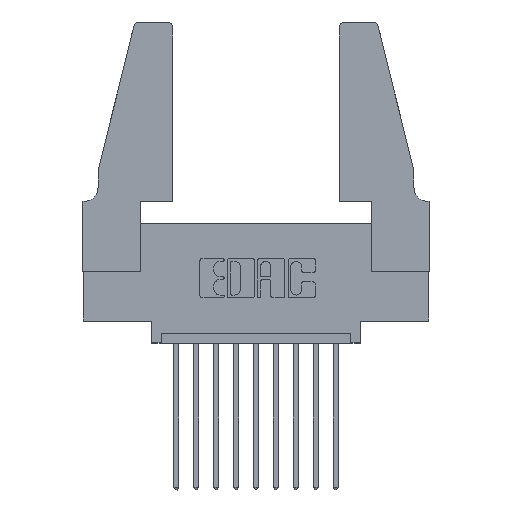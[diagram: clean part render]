
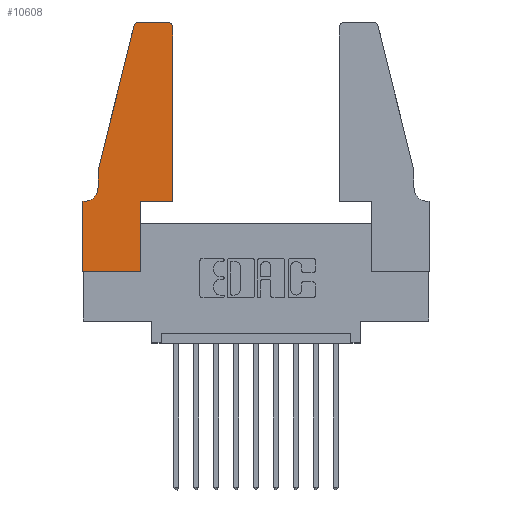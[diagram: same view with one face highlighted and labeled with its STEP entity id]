
A CAD part, top view. The second image highlights one B-rep face of the part: STEP entity #10608.
In plain terms, the highlighted planar face has unit normal (0, 0, 1).
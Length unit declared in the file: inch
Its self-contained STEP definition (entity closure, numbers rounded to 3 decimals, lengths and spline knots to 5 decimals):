
#60 = LINE ( 'NONE', #7379, #5006 ) ;
#385 = CARTESIAN_POINT ( 'NONE',  ( 0.0055, 0.42, 0.37 ) ) ;
#438 = DIRECTION ( 'NONE',  ( 0., -1., 0. ) ) ;
#533 = LINE ( 'NONE', #12607, #9063 ) ;
#755 = ORIENTED_EDGE ( 'NONE', *, *, #12746, .T. ) ;
#870 = LINE ( 'NONE', #3170, #8243 ) ;
#896 = CIRCLE ( 'NONE', #7988, 0.03 ) ;
#925 = CARTESIAN_POINT ( 'NONE',  ( 0.0755, 0.5, 0.37 ) ) ;
#957 = EDGE_CURVE ( 'NONE', #6256, #11347, #60, .T. ) ;
#1126 = AXIS2_PLACEMENT_3D ( 'NONE', #10207, #1919, #12230 ) ;
#1200 = EDGE_CURVE ( 'NONE', #6721, #6256, #12847, .T. ) ;
#1493 = VERTEX_POINT ( 'NONE', #5527 ) ;
#1587 = CARTESIAN_POINT ( 'NONE',  ( 0.2865, 0.35, 0.37 ) ) ;
#1686 = EDGE_CURVE ( 'NONE', #3656, #1854, #870, .T. ) ;
#1854 = VERTEX_POINT ( 'NONE', #8184 ) ;
#1919 = DIRECTION ( 'NONE',  ( 0., 0., 1. ) ) ;
#2016 = ORIENTED_EDGE ( 'NONE', *, *, #1200, .T. ) ;
#2304 = DIRECTION ( 'NONE',  ( 0., 1., 0. ) ) ;
#2331 = CARTESIAN_POINT ( 'NONE',  ( 0., 0.35, 0.37 ) ) ;
#2590 = CARTESIAN_POINT ( 'NONE',  ( 0.4505, 0.35, 0.37 ) ) ;
#2625 = DIRECTION ( 'NONE',  ( 0., 0., 1. ) ) ;
#2951 = AXIS2_PLACEMENT_3D ( 'NONE', #2331, #11775, #6443 ) ;
#2980 = LINE ( 'NONE', #12002, #6935 ) ;
#3170 = CARTESIAN_POINT ( 'NONE',  ( 0.2605, 1.25, 0.37 ) ) ;
#3343 = CIRCLE ( 'NONE', #1126, 0.03 ) ;
#3351 = DIRECTION ( 'NONE',  ( 1., 0., 0. ) ) ;
#3488 = CARTESIAN_POINT ( 'NONE',  ( 0.0755, 0.42, 0.37 ) ) ;
#3578 = VERTEX_POINT ( 'NONE', #925 ) ;
#3620 = ORIENTED_EDGE ( 'NONE', *, *, #957, .T. ) ;
#3642 = VERTEX_POINT ( 'NONE', #6385 ) ;
#3656 = VERTEX_POINT ( 'NONE', #6252 ) ;
#3939 = CARTESIAN_POINT ( 'NONE',  ( 0.0755, 0.5, 0.37 ) ) ;
#4264 = CARTESIAN_POINT ( 'NONE',  ( 0., 0.35, 0.37 ) ) ;
#4379 = ORIENTED_EDGE ( 'NONE', *, *, #6193, .T. ) ;
#4817 = DIRECTION ( 'NONE',  ( 1., 0., 0. ) ) ;
#4852 = DIRECTION ( 'NONE',  ( 1., 0., 0. ) ) ;
#4925 = ORIENTED_EDGE ( 'NONE', *, *, #7221, .T. ) ;
#4963 = LINE ( 'NONE', #3939, #8701 ) ;
#4997 = DIRECTION ( 'NONE',  ( -0.239, -0.971, 0. ) ) ;
#5006 = VECTOR ( 'NONE', #2304, 39.37008 ) ;
#5093 = LINE ( 'NONE', #10702, #11446 ) ;
#5118 = EDGE_CURVE ( 'NONE', #1854, #7460, #896, .T. ) ;
#5527 = CARTESIAN_POINT ( 'NONE',  ( 0.0055, 0.35, 0.37 ) ) ;
#5641 = CARTESIAN_POINT ( 'NONE',  ( 0., 0., 0.37 ) ) ;
#5707 = LINE ( 'NONE', #1587, #8457 ) ;
#5742 = DIRECTION ( 'NONE',  ( -1., 0., 0. ) ) ;
#5833 = DIRECTION ( 'NONE',  ( 0., 1., 0. ) ) ;
#6193 = EDGE_CURVE ( 'NONE', #3578, #10670, #6798, .T. ) ;
#6252 = CARTESIAN_POINT ( 'NONE',  ( 0.4205, 1.25, 0.37 ) ) ;
#6256 = VERTEX_POINT ( 'NONE', #9114 ) ;
#6266 = EDGE_CURVE ( 'NONE', #11347, #3656, #3343, .T. ) ;
#6385 = CARTESIAN_POINT ( 'NONE',  ( 0.2865, 0., 0.37 ) ) ;
#6443 = DIRECTION ( 'NONE',  ( 1., 0., 0. ) ) ;
#6455 = EDGE_CURVE ( 'NONE', #1493, #6478, #533, .T. ) ;
#6478 = VERTEX_POINT ( 'NONE', #4264 ) ;
#6567 = ORIENTED_EDGE ( 'NONE', *, *, #12568, .T. ) ;
#6625 = PLANE ( 'NONE',  #2951 ) ;
#6660 = AXIS2_PLACEMENT_3D ( 'NONE', #385, #11977, #5742 ) ;
#6721 = VERTEX_POINT ( 'NONE', #13373 ) ;
#6798 = LINE ( 'NONE', #10301, #12992 ) ;
#6805 = VECTOR ( 'NONE', #4817, 39.37008 ) ;
#6935 = VECTOR ( 'NONE', #438, 39.37008 ) ;
#7148 = CARTESIAN_POINT ( 'NONE',  ( 0.25487, 1.22718, 0.37 ) ) ;
#7221 = EDGE_CURVE ( 'NONE', #6478, #9861, #2980, .T. ) ;
#7379 = CARTESIAN_POINT ( 'NONE',  ( 0.4505, 0.35, 0.37 ) ) ;
#7460 = VERTEX_POINT ( 'NONE', #7148 ) ;
#7537 = CARTESIAN_POINT ( 'NONE',  ( 0.4505, 1.22, 0.37 ) ) ;
#7988 = AXIS2_PLACEMENT_3D ( 'NONE', #8989, #2625, #4852 ) ;
#8184 = CARTESIAN_POINT ( 'NONE',  ( 0.284, 1.25, 0.37 ) ) ;
#8218 = CIRCLE ( 'NONE', #6660, 0.07 ) ;
#8243 = VECTOR ( 'NONE', #8250, 39.37008 ) ;
#8250 = DIRECTION ( 'NONE',  ( -1., 0., 0. ) ) ;
#8457 = VECTOR ( 'NONE', #5833, 39.37008 ) ;
#8528 = EDGE_CURVE ( 'NONE', #9861, #3642, #5093, .T. ) ;
#8701 = VECTOR ( 'NONE', #4997, 39.37008 ) ;
#8989 = CARTESIAN_POINT ( 'NONE',  ( 0.284, 1.22, 0.37 ) ) ;
#9063 = VECTOR ( 'NONE', #12506, 39.37008 ) ;
#9114 = CARTESIAN_POINT ( 'NONE',  ( 0.4505, 0.35, 0.37 ) ) ;
#9170 = ORIENTED_EDGE ( 'NONE', *, *, #5118, .T. ) ;
#9861 = VERTEX_POINT ( 'NONE', #5641 ) ;
#9950 = EDGE_CURVE ( 'NONE', #3642, #6721, #5707, .T. ) ;
#10207 = CARTESIAN_POINT ( 'NONE',  ( 0.4205, 1.22, 0.37 ) ) ;
#10290 = ORIENTED_EDGE ( 'NONE', *, *, #1686, .T. ) ;
#10301 = CARTESIAN_POINT ( 'NONE',  ( 0.0755, 0.5, 0.37 ) ) ;
#10608 = ADVANCED_FACE ( 'NONE', ( #12232 ), #6625, .T. ) ;
#10670 = VERTEX_POINT ( 'NONE', #3488 ) ;
#10702 = CARTESIAN_POINT ( 'NONE',  ( 0., 0., 0.37 ) ) ;
#11019 = ORIENTED_EDGE ( 'NONE', *, *, #8528, .T. ) ;
#11026 = EDGE_LOOP ( 'NONE', ( #10290, #9170, #755, #4379, #6567, #12334, #4925, #11019, #12866, #2016, #3620, #13528 ) ) ;
#11347 = VERTEX_POINT ( 'NONE', #7537 ) ;
#11446 = VECTOR ( 'NONE', #3351, 39.37008 ) ;
#11775 = DIRECTION ( 'NONE',  ( 0., 0., 1. ) ) ;
#11977 = DIRECTION ( 'NONE',  ( 0., 0., -1. ) ) ;
#12002 = CARTESIAN_POINT ( 'NONE',  ( 0., 0., 0.37 ) ) ;
#12230 = DIRECTION ( 'NONE',  ( 1., 0., 0. ) ) ;
#12232 = FACE_OUTER_BOUND ( 'NONE', #11026, .T. ) ;
#12276 = DIRECTION ( 'NONE',  ( 0., -1., 0. ) ) ;
#12334 = ORIENTED_EDGE ( 'NONE', *, *, #6455, .T. ) ;
#12506 = DIRECTION ( 'NONE',  ( -1., 0., 0. ) ) ;
#12568 = EDGE_CURVE ( 'NONE', #10670, #1493, #8218, .T. ) ;
#12607 = CARTESIAN_POINT ( 'NONE',  ( 0.0755, 0.35, 0.37 ) ) ;
#12746 = EDGE_CURVE ( 'NONE', #7460, #3578, #4963, .T. ) ;
#12847 = LINE ( 'NONE', #2590, #6805 ) ;
#12866 = ORIENTED_EDGE ( 'NONE', *, *, #9950, .T. ) ;
#12992 = VECTOR ( 'NONE', #12276, 39.37008 ) ;
#13373 = CARTESIAN_POINT ( 'NONE',  ( 0.2865, 0.35, 0.37 ) ) ;
#13528 = ORIENTED_EDGE ( 'NONE', *, *, #6266, .T. ) ;
